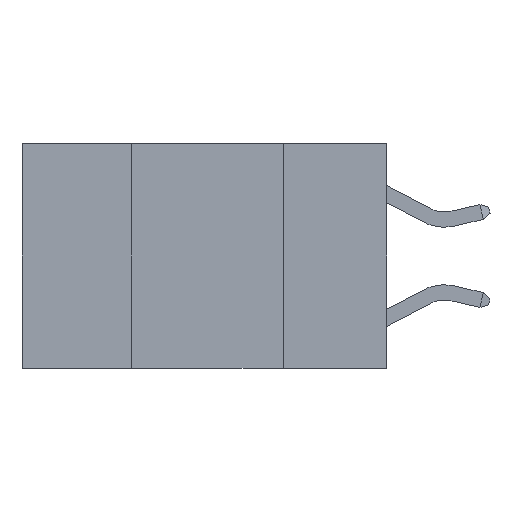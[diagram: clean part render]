
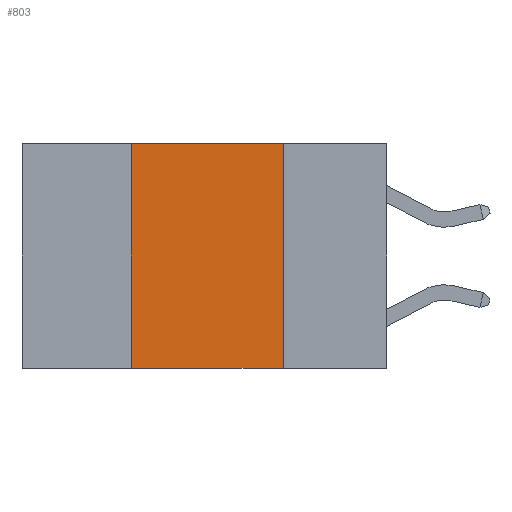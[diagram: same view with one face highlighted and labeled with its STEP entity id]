
A CAD part, left-side view. The second image highlights one B-rep face of the part: STEP entity #803.
In plain terms, the highlighted planar face has unit normal (-1, 0, 0).
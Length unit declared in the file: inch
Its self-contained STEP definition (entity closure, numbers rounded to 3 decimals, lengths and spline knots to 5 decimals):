
#8 = DIRECTION ( 'NONE',  ( 0., -1., 0. ) ) ;
#803 = ADVANCED_FACE ( 'NONE', ( #6454 ), #1028, .F. ) ;
#1028 = PLANE ( 'NONE',  #7910 ) ;
#2225 = DIRECTION ( 'NONE',  ( 1., 0., 0. ) ) ;
#2487 = CARTESIAN_POINT ( 'NONE',  ( 0., 0.6, 0. ) ) ;
#2807 = ORIENTED_EDGE ( 'NONE', *, *, #8709, .T. ) ;
#2910 = CARTESIAN_POINT ( 'NONE',  ( 0., 0.17, 0. ) ) ;
#3131 = VERTEX_POINT ( 'NONE', #2910 ) ;
#3194 = VERTEX_POINT ( 'NONE', #12629 ) ;
#3524 = EDGE_CURVE ( 'NONE', #3194, #3131, #9163, .T. ) ;
#5589 = ORIENTED_EDGE ( 'NONE', *, *, #9515, .F. ) ;
#5769 = VERTEX_POINT ( 'NONE', #6168 ) ;
#5950 = LINE ( 'NONE', #12641, #15139 ) ;
#5982 = VECTOR ( 'NONE', #14457, 39.37008 ) ;
#6168 = CARTESIAN_POINT ( 'NONE',  ( 0., 0.42, -0.37 ) ) ;
#6454 = FACE_OUTER_BOUND ( 'NONE', #12504, .T. ) ;
#6775 = VECTOR ( 'NONE', #8, 39.37008 ) ;
#7162 = CARTESIAN_POINT ( 'NONE',  ( 0., 0.6, -0.37 ) ) ;
#7910 = AXIS2_PLACEMENT_3D ( 'NONE', #9380, #2225, #10607 ) ;
#8245 = LINE ( 'NONE', #14617, #14259 ) ;
#8647 = DIRECTION ( 'NONE',  ( 0., 0., 1. ) ) ;
#8709 = EDGE_CURVE ( 'NONE', #5769, #8989, #12789, .T. ) ;
#8989 = VERTEX_POINT ( 'NONE', #14848 ) ;
#9163 = LINE ( 'NONE', #2487, #5982 ) ;
#9380 = CARTESIAN_POINT ( 'NONE',  ( 0., 0.6, 0. ) ) ;
#9515 = EDGE_CURVE ( 'NONE', #5769, #3194, #8245, .T. ) ;
#10607 = DIRECTION ( 'NONE',  ( 0., 0., -1. ) ) ;
#11134 = EDGE_CURVE ( 'NONE', #3131, #8989, #5950, .T. ) ;
#11228 = ORIENTED_EDGE ( 'NONE', *, *, #11134, .F. ) ;
#12504 = EDGE_LOOP ( 'NONE', ( #11228, #14776, #5589, #2807 ) ) ;
#12629 = CARTESIAN_POINT ( 'NONE',  ( 0., 0.42, 0. ) ) ;
#12641 = CARTESIAN_POINT ( 'NONE',  ( 0., 0.17, 0. ) ) ;
#12789 = LINE ( 'NONE', #7162, #6775 ) ;
#13867 = DIRECTION ( 'NONE',  ( 0., 0., -1. ) ) ;
#14259 = VECTOR ( 'NONE', #8647, 39.37008 ) ;
#14457 = DIRECTION ( 'NONE',  ( 0., -1., 0. ) ) ;
#14617 = CARTESIAN_POINT ( 'NONE',  ( 0., 0.42, 0. ) ) ;
#14776 = ORIENTED_EDGE ( 'NONE', *, *, #3524, .F. ) ;
#14848 = CARTESIAN_POINT ( 'NONE',  ( 0., 0.17, -0.37 ) ) ;
#15139 = VECTOR ( 'NONE', #13867, 39.37008 ) ;
